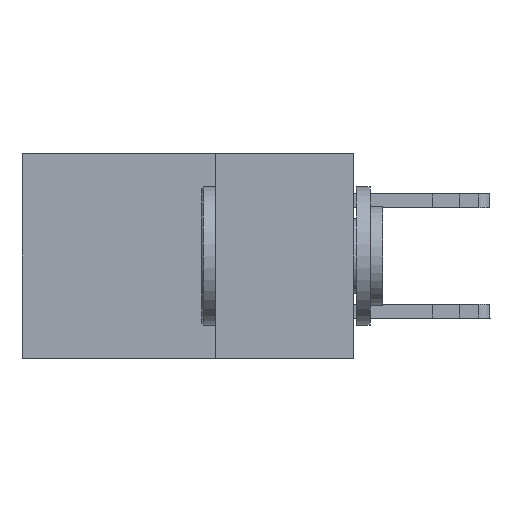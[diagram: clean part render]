
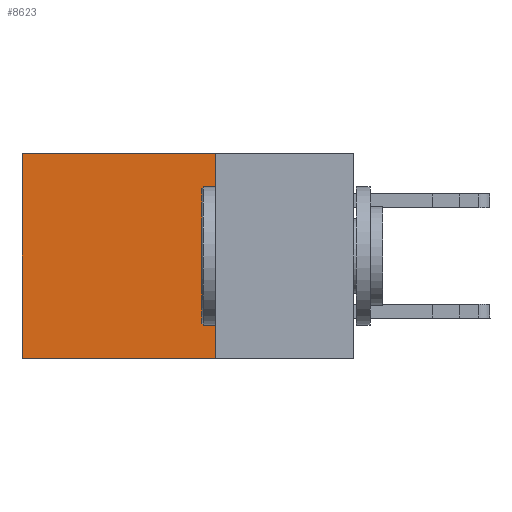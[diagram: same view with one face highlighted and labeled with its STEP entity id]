
A CAD part, left-side view. The second image highlights one B-rep face of the part: STEP entity #8623.
In plain terms, the highlighted planar face has unit normal (-1, 0, 0).
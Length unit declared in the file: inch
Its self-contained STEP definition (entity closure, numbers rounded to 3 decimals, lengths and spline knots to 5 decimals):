
#124 = EDGE_LOOP ( 'NONE', ( #15901, #10947, #9849, #17232 ) ) ;
#525 = AXIS2_PLACEMENT_3D ( 'NONE', #17243, #2141, #12186 ) ;
#1683 = DIRECTION ( 'NONE',  ( 0., 0., -1. ) ) ;
#2141 = DIRECTION ( 'NONE',  ( 1., 0., 0. ) ) ;
#2503 = EDGE_CURVE ( 'NONE', #15745, #8086, #9567, .T. ) ;
#3548 = EDGE_CURVE ( 'NONE', #15745, #4092, #13676, .T. ) ;
#3791 = VECTOR ( 'NONE', #17796, 39.37008 ) ;
#3830 = FACE_OUTER_BOUND ( 'NONE', #124, .T. ) ;
#3974 = EDGE_CURVE ( 'NONE', #4092, #15368, #15220, .T. ) ;
#4092 = VERTEX_POINT ( 'NONE', #16881 ) ;
#4123 = CARTESIAN_POINT ( 'NONE',  ( 0.2875, 0.25, 0. ) ) ;
#4147 = DIRECTION ( 'NONE',  ( 0., 1., 0. ) ) ;
#4153 = CARTESIAN_POINT ( 'NONE',  ( 0.2875, 0.25, 0. ) ) ;
#4892 = CARTESIAN_POINT ( 'NONE',  ( 0.2875, 0.25, 0. ) ) ;
#5325 = DIRECTION ( 'NONE',  ( 0., 1., 0. ) ) ;
#6409 = EDGE_CURVE ( 'NONE', #8086, #15368, #6734, .T. ) ;
#6734 = LINE ( 'NONE', #13633, #13992 ) ;
#7205 = CARTESIAN_POINT ( 'NONE',  ( 0.2875, 0.6, -0.37 ) ) ;
#8086 = VERTEX_POINT ( 'NONE', #10605 ) ;
#8623 = ADVANCED_FACE ( 'NONE', ( #3830 ), #10875, .F. ) ;
#9567 = LINE ( 'NONE', #4153, #12282 ) ;
#9849 = ORIENTED_EDGE ( 'NONE', *, *, #2503, .F. ) ;
#10605 = CARTESIAN_POINT ( 'NONE',  ( 0.2875, 0.25, -0.37 ) ) ;
#10875 = PLANE ( 'NONE',  #525 ) ;
#10947 = ORIENTED_EDGE ( 'NONE', *, *, #6409, .F. ) ;
#12186 = DIRECTION ( 'NONE',  ( 0., 0., -1. ) ) ;
#12282 = VECTOR ( 'NONE', #1683, 39.37008 ) ;
#13633 = CARTESIAN_POINT ( 'NONE',  ( 0.2875, 0.25, -0.37 ) ) ;
#13676 = LINE ( 'NONE', #4123, #16621 ) ;
#13992 = VECTOR ( 'NONE', #5325, 39.37008 ) ;
#15220 = LINE ( 'NONE', #17683, #3791 ) ;
#15368 = VERTEX_POINT ( 'NONE', #7205 ) ;
#15745 = VERTEX_POINT ( 'NONE', #4892 ) ;
#15901 = ORIENTED_EDGE ( 'NONE', *, *, #3974, .T. ) ;
#16621 = VECTOR ( 'NONE', #4147, 39.37008 ) ;
#16881 = CARTESIAN_POINT ( 'NONE',  ( 0.2875, 0.6, 0. ) ) ;
#17232 = ORIENTED_EDGE ( 'NONE', *, *, #3548, .T. ) ;
#17243 = CARTESIAN_POINT ( 'NONE',  ( 0.2875, 0.25, 0. ) ) ;
#17683 = CARTESIAN_POINT ( 'NONE',  ( 0.2875, 0.6, 0. ) ) ;
#17796 = DIRECTION ( 'NONE',  ( 0., 0., -1. ) ) ;
